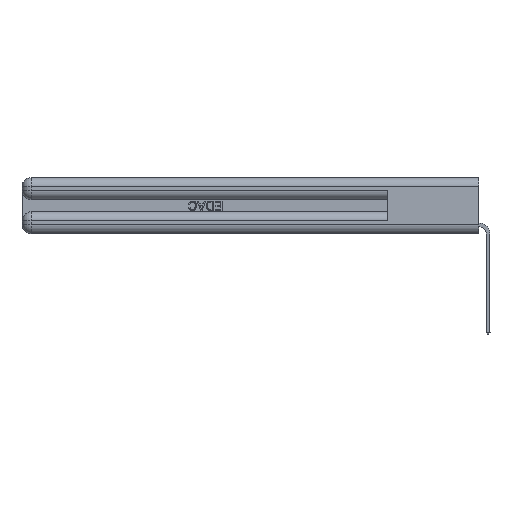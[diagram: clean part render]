
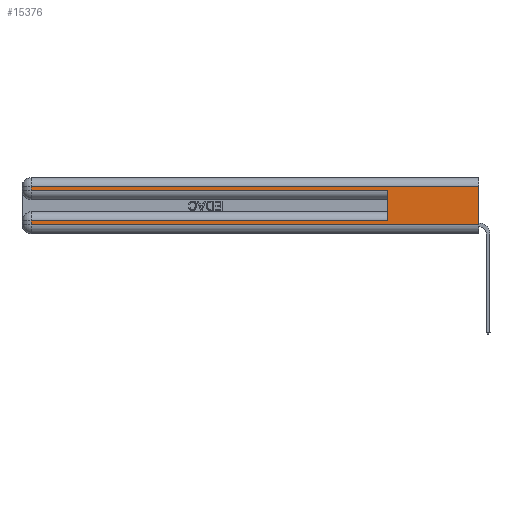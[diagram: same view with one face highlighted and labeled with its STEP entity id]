
A CAD part, left-side view. The second image highlights one B-rep face of the part: STEP entity #15376.
In plain terms, the highlighted planar face has unit normal (-1, 0, 0).
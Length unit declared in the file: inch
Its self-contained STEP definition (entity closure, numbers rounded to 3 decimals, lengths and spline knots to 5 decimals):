
#120 = DIRECTION ( 'NONE',  ( 0., 0., -1. ) ) ;
#1695 = CARTESIAN_POINT ( 'NONE',  ( 0., 0., 0.085 ) ) ;
#2014 = EDGE_CURVE ( 'NONE', #19855, #16433, #6564, .T. ) ;
#2061 = LINE ( 'NONE', #17498, #8299 ) ;
#2352 = VERTEX_POINT ( 'NONE', #7756 ) ;
#3043 = AXIS2_PLACEMENT_3D ( 'NONE', #18755, #12624, #120 ) ;
#3426 = EDGE_CURVE ( 'NONE', #5503, #19855, #15626, .T. ) ;
#3725 = VECTOR ( 'NONE', #3989, 39.37008 ) ;
#3749 = CARTESIAN_POINT ( 'NONE',  ( 0., 0., 0.31 ) ) ;
#3989 = DIRECTION ( 'NONE',  ( 0., 0., -1. ) ) ;
#5231 = ORIENTED_EDGE ( 'NONE', *, *, #24322, .F. ) ;
#5503 = VERTEX_POINT ( 'NONE', #22349 ) ;
#5574 = ORIENTED_EDGE ( 'NONE', *, *, #10418, .T. ) ;
#6274 = CARTESIAN_POINT ( 'NONE',  ( 0., 0.6, 0.085 ) ) ;
#6564 = LINE ( 'NONE', #17142, #11451 ) ;
#6757 = DIRECTION ( 'NONE',  ( 0., -1., 0. ) ) ;
#7115 = DIRECTION ( 'NONE',  ( 0., -1., 0. ) ) ;
#7202 = LINE ( 'NONE', #1695, #12073 ) ;
#7756 = CARTESIAN_POINT ( 'NONE',  ( 0., 2.94, 0.31 ) ) ;
#8299 = VECTOR ( 'NONE', #7115, 39.37008 ) ;
#8547 = DIRECTION ( 'NONE',  ( 0., 0., 1. ) ) ;
#8699 = CARTESIAN_POINT ( 'NONE',  ( 0., 0., 0.31 ) ) ;
#9285 = LINE ( 'NONE', #14414, #3725 ) ;
#9653 = VERTEX_POINT ( 'NONE', #3749 ) ;
#9824 = ORIENTED_EDGE ( 'NONE', *, *, #11819, .F. ) ;
#10073 = VECTOR ( 'NONE', #18250, 39.37008 ) ;
#10418 = EDGE_CURVE ( 'NONE', #24922, #5503, #7202, .T. ) ;
#11451 = VECTOR ( 'NONE', #6757, 39.37008 ) ;
#11819 = EDGE_CURVE ( 'NONE', #24922, #23151, #12873, .T. ) ;
#12073 = VECTOR ( 'NONE', #20481, 39.37008 ) ;
#12624 = DIRECTION ( 'NONE',  ( 1., 0., 0. ) ) ;
#12873 = LINE ( 'NONE', #23077, #24551 ) ;
#13217 = EDGE_CURVE ( 'NONE', #16469, #23151, #2061, .T. ) ;
#13408 = ORIENTED_EDGE ( 'NONE', *, *, #21578, .T. ) ;
#13752 = ORIENTED_EDGE ( 'NONE', *, *, #2014, .T. ) ;
#14414 = CARTESIAN_POINT ( 'NONE',  ( 0., 0., 0.37 ) ) ;
#15376 = ADVANCED_FACE ( 'NONE', ( #23104 ), #25055, .F. ) ;
#15626 = LINE ( 'NONE', #24368, #10073 ) ;
#15649 = VECTOR ( 'NONE', #19106, 39.37008 ) ;
#15730 = VECTOR ( 'NONE', #22845, 39.37008 ) ;
#16433 = VERTEX_POINT ( 'NONE', #23264 ) ;
#16469 = VERTEX_POINT ( 'NONE', #17222 ) ;
#17142 = CARTESIAN_POINT ( 'NONE',  ( 0., 0., 0.06 ) ) ;
#17222 = CARTESIAN_POINT ( 'NONE',  ( 0., 2.94, 0.285 ) ) ;
#17498 = CARTESIAN_POINT ( 'NONE',  ( 0., 0., 0.285 ) ) ;
#18250 = DIRECTION ( 'NONE',  ( 0., 0., -1. ) ) ;
#18638 = ORIENTED_EDGE ( 'NONE', *, *, #3426, .T. ) ;
#18755 = CARTESIAN_POINT ( 'NONE',  ( 0., 0., 0.37 ) ) ;
#18808 = CARTESIAN_POINT ( 'NONE',  ( 0., 2.94, 0.37 ) ) ;
#19106 = DIRECTION ( 'NONE',  ( 0., 1., 0. ) ) ;
#19855 = VERTEX_POINT ( 'NONE', #23757 ) ;
#20212 = EDGE_CURVE ( 'NONE', #2352, #16469, #21884, .T. ) ;
#20264 = ORIENTED_EDGE ( 'NONE', *, *, #13217, .T. ) ;
#20481 = DIRECTION ( 'NONE',  ( 0., 1., 0. ) ) ;
#20745 = EDGE_LOOP ( 'NONE', ( #5231, #13408, #24411, #20264, #9824, #5574, #18638, #13752 ) ) ;
#21578 = EDGE_CURVE ( 'NONE', #9653, #2352, #26027, .T. ) ;
#21884 = LINE ( 'NONE', #18808, #15730 ) ;
#22349 = CARTESIAN_POINT ( 'NONE',  ( 0., 2.94, 0.085 ) ) ;
#22355 = CARTESIAN_POINT ( 'NONE',  ( 0., 0.6, 0.285 ) ) ;
#22845 = DIRECTION ( 'NONE',  ( 0., 0., -1. ) ) ;
#23077 = CARTESIAN_POINT ( 'NONE',  ( 0., 0.6, 0.145 ) ) ;
#23104 = FACE_OUTER_BOUND ( 'NONE', #20745, .T. ) ;
#23151 = VERTEX_POINT ( 'NONE', #22355 ) ;
#23264 = CARTESIAN_POINT ( 'NONE',  ( 0., 0., 0.06 ) ) ;
#23757 = CARTESIAN_POINT ( 'NONE',  ( 0., 2.94, 0.06 ) ) ;
#24322 = EDGE_CURVE ( 'NONE', #9653, #16433, #9285, .T. ) ;
#24368 = CARTESIAN_POINT ( 'NONE',  ( 0., 2.94, 0.37 ) ) ;
#24411 = ORIENTED_EDGE ( 'NONE', *, *, #20212, .T. ) ;
#24551 = VECTOR ( 'NONE', #8547, 39.37008 ) ;
#24922 = VERTEX_POINT ( 'NONE', #6274 ) ;
#25055 = PLANE ( 'NONE',  #3043 ) ;
#26027 = LINE ( 'NONE', #8699, #15649 ) ;
